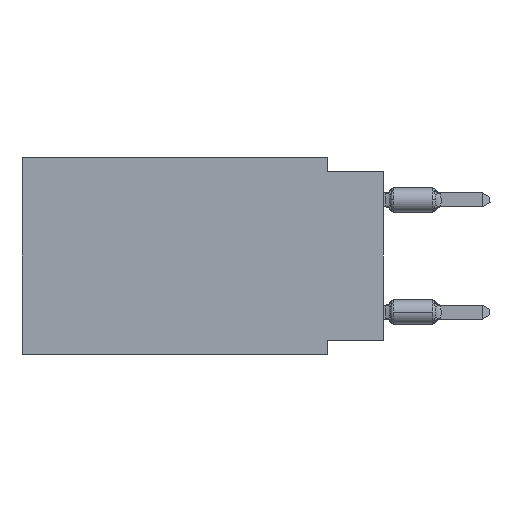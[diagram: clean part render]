
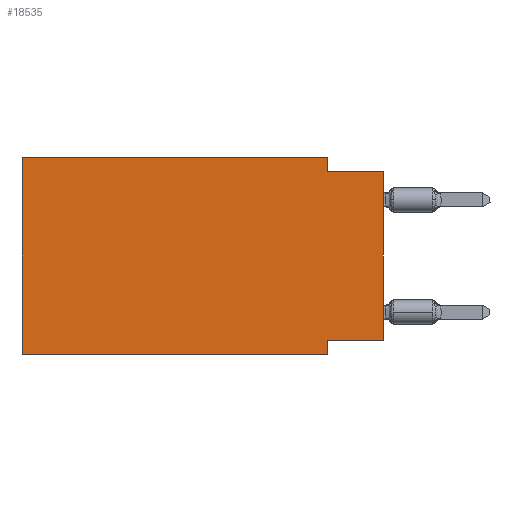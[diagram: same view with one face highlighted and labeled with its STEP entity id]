
A CAD part, left-side view. The second image highlights one B-rep face of the part: STEP entity #18535.
In plain terms, the highlighted planar face has unit normal (-1, 0, 0).
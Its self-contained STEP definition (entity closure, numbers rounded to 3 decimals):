
#1016 = ORIENTED_EDGE ( 'NONE', *, *, #26074, .F. ) ;
#1098 = ORIENTED_EDGE ( 'NONE', *, *, #27018, .F. ) ;
#1708 = CARTESIAN_POINT ( 'NONE',  ( 0., 2.54, 0. ) ) ;
#1755 = LINE ( 'NONE', #6594, #28320 ) ;
#2085 = FACE_OUTER_BOUND ( 'NONE', #10570, .T. ) ;
#2916 = EDGE_CURVE ( 'NONE', #19221, #3977, #15741, .T. ) ;
#3073 = EDGE_CURVE ( 'NONE', #15968, #10416, #7731, .T. ) ;
#3977 = VERTEX_POINT ( 'NONE', #7655 ) ;
#4110 = CARTESIAN_POINT ( 'NONE',  ( 0., 0., -0.635 ) ) ;
#4980 = VECTOR ( 'NONE', #17289, 1000. ) ;
#5499 = CARTESIAN_POINT ( 'NONE',  ( 0., 0., -8.255 ) ) ;
#5645 = LINE ( 'NONE', #5499, #7734 ) ;
#6551 = LINE ( 'NONE', #1708, #21475 ) ;
#6594 = CARTESIAN_POINT ( 'NONE',  ( 0., 2.54, -8.89 ) ) ;
#6611 = PLANE ( 'NONE',  #16215 ) ;
#6629 = VECTOR ( 'NONE', #13097, 1000. ) ;
#6843 = VECTOR ( 'NONE', #21057, 1000. ) ;
#6962 = DIRECTION ( 'NONE',  ( 0., -1., 0. ) ) ;
#7230 = ORIENTED_EDGE ( 'NONE', *, *, #2916, .T. ) ;
#7655 = CARTESIAN_POINT ( 'NONE',  ( 0., 2.54, -8.89 ) ) ;
#7731 = LINE ( 'NONE', #12597, #4980 ) ;
#7734 = VECTOR ( 'NONE', #24632, 1000. ) ;
#8020 = CARTESIAN_POINT ( 'NONE',  ( 0., 2.54, -0.635 ) ) ;
#8134 = EDGE_CURVE ( 'NONE', #10601, #26167, #20974, .T. ) ;
#9219 = DIRECTION ( 'NONE',  ( 0., 0., 1. ) ) ;
#10037 = ORIENTED_EDGE ( 'NONE', *, *, #8134, .T. ) ;
#10416 = VERTEX_POINT ( 'NONE', #16665 ) ;
#10426 = VERTEX_POINT ( 'NONE', #8020 ) ;
#10570 = EDGE_LOOP ( 'NONE', ( #10037, #29547, #13573, #17547, #1098, #7230, #16307, #1016 ) ) ;
#10601 = VERTEX_POINT ( 'NONE', #30595 ) ;
#10899 = LINE ( 'NONE', #17789, #6629 ) ;
#10950 = CARTESIAN_POINT ( 'NONE',  ( 0., 2.54, -8.255 ) ) ;
#11271 = DIRECTION ( 'NONE',  ( 0., 0., -1. ) ) ;
#11334 = DIRECTION ( 'NONE',  ( 0., 0., -1. ) ) ;
#12588 = VERTEX_POINT ( 'NONE', #10950 ) ;
#12597 = CARTESIAN_POINT ( 'NONE',  ( 0., 16.383, 0. ) ) ;
#13097 = DIRECTION ( 'NONE',  ( 0., 0., 1. ) ) ;
#13411 = EDGE_CURVE ( 'NONE', #12588, #3977, #1755, .T. ) ;
#13573 = ORIENTED_EDGE ( 'NONE', *, *, #29850, .F. ) ;
#13839 = DIRECTION ( 'NONE',  ( 1., 0., 0. ) ) ;
#15741 = LINE ( 'NONE', #25316, #19984 ) ;
#15968 = VERTEX_POINT ( 'NONE', #27437 ) ;
#16161 = DIRECTION ( 'NONE',  ( 0., 0., -1. ) ) ;
#16215 = AXIS2_PLACEMENT_3D ( 'NONE', #28432, #13839, #11334 ) ;
#16307 = ORIENTED_EDGE ( 'NONE', *, *, #13411, .F. ) ;
#16665 = CARTESIAN_POINT ( 'NONE',  ( 0., 2.54, 0. ) ) ;
#17289 = DIRECTION ( 'NONE',  ( 0., -1., 0. ) ) ;
#17547 = ORIENTED_EDGE ( 'NONE', *, *, #3073, .F. ) ;
#17789 = CARTESIAN_POINT ( 'NONE',  ( 0., 16.383, 0. ) ) ;
#18259 = CARTESIAN_POINT ( 'NONE',  ( 0., 16.383, -8.89 ) ) ;
#18535 = ADVANCED_FACE ( 'NONE', ( #2085 ), #6611, .F. ) ;
#18609 = CARTESIAN_POINT ( 'NONE',  ( 0., 0., 0. ) ) ;
#19221 = VERTEX_POINT ( 'NONE', #18259 ) ;
#19667 = VECTOR ( 'NONE', #9219, 1000. ) ;
#19706 = EDGE_CURVE ( 'NONE', #10426, #26167, #30304, .T. ) ;
#19984 = VECTOR ( 'NONE', #6962, 1000. ) ;
#20974 = LINE ( 'NONE', #18609, #19667 ) ;
#21057 = DIRECTION ( 'NONE',  ( 0., -1., 0. ) ) ;
#21475 = VECTOR ( 'NONE', #11271, 1000. ) ;
#24632 = DIRECTION ( 'NONE',  ( 0., 1., 0. ) ) ;
#25316 = CARTESIAN_POINT ( 'NONE',  ( 0., 16.383, -8.89 ) ) ;
#26074 = EDGE_CURVE ( 'NONE', #10601, #12588, #5645, .T. ) ;
#26167 = VERTEX_POINT ( 'NONE', #30410 ) ;
#27018 = EDGE_CURVE ( 'NONE', #19221, #15968, #10899, .T. ) ;
#27437 = CARTESIAN_POINT ( 'NONE',  ( 0., 16.383, 0. ) ) ;
#28320 = VECTOR ( 'NONE', #16161, 1000. ) ;
#28432 = CARTESIAN_POINT ( 'NONE',  ( 0., 16.383, 0. ) ) ;
#29547 = ORIENTED_EDGE ( 'NONE', *, *, #19706, .F. ) ;
#29850 = EDGE_CURVE ( 'NONE', #10416, #10426, #6551, .T. ) ;
#30304 = LINE ( 'NONE', #4110, #6843 ) ;
#30410 = CARTESIAN_POINT ( 'NONE',  ( 0., 0., -0.635 ) ) ;
#30595 = CARTESIAN_POINT ( 'NONE',  ( 0., 0., -8.255 ) ) ;
